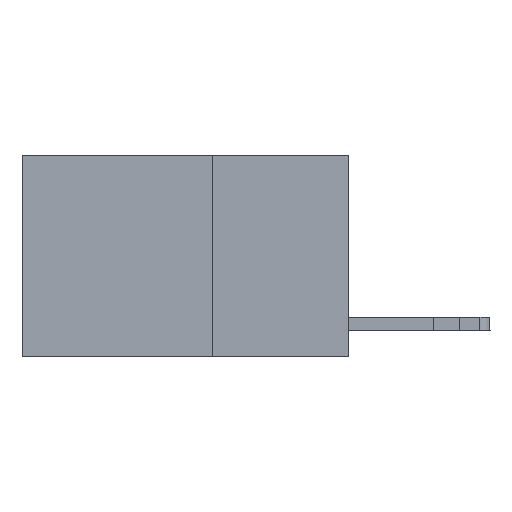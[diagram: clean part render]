
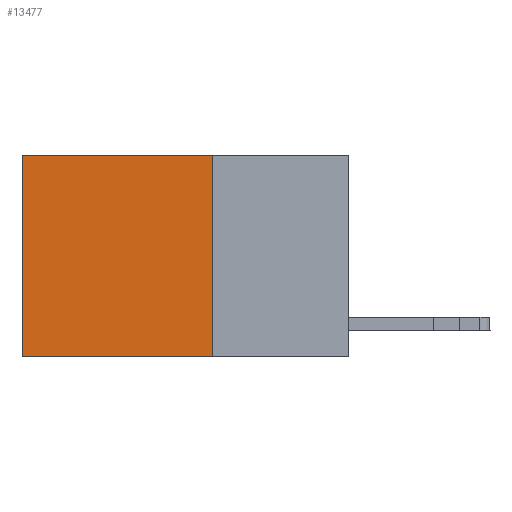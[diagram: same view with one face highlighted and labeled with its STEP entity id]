
A CAD part, left-side view. The second image highlights one B-rep face of the part: STEP entity #13477.
In plain terms, the highlighted planar face has unit normal (-1, 0, 0).
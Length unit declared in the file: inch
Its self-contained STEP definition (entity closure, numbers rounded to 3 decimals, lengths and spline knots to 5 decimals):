
#238 = CARTESIAN_POINT ( 'NONE',  ( 0.2625, 0.25, 0. ) ) ;
#240 = EDGE_CURVE ( 'NONE', #11728, #13563, #1599, .T. ) ;
#312 = DIRECTION ( 'NONE',  ( 0., 1., 0. ) ) ;
#482 = CARTESIAN_POINT ( 'NONE',  ( 0.2625, 0.6, 0. ) ) ;
#1485 = CARTESIAN_POINT ( 'NONE',  ( 0.2625, 0.25, -0.37 ) ) ;
#1599 = LINE ( 'NONE', #238, #4225 ) ;
#1971 = EDGE_LOOP ( 'NONE', ( #6994, #4688, #11610, #4409 ) ) ;
#4225 = VECTOR ( 'NONE', #13437, 39.37008 ) ;
#4297 = LINE ( 'NONE', #482, #6034 ) ;
#4409 = ORIENTED_EDGE ( 'NONE', *, *, #16206, .T. ) ;
#4688 = ORIENTED_EDGE ( 'NONE', *, *, #7152, .F. ) ;
#5557 = LINE ( 'NONE', #13019, #9569 ) ;
#5645 = DIRECTION ( 'NONE',  ( 0., 0., -1. ) ) ;
#6034 = VECTOR ( 'NONE', #5645, 39.37008 ) ;
#6400 = DIRECTION ( 'NONE',  ( 0., 0., -1. ) ) ;
#6994 = ORIENTED_EDGE ( 'NONE', *, *, #8410, .T. ) ;
#7145 = LINE ( 'NONE', #9414, #8613 ) ;
#7152 = EDGE_CURVE ( 'NONE', #13563, #13958, #5557, .T. ) ;
#7856 = CARTESIAN_POINT ( 'NONE',  ( 0.2625, 0.25, 0. ) ) ;
#8410 = EDGE_CURVE ( 'NONE', #10838, #13958, #4297, .T. ) ;
#8546 = CARTESIAN_POINT ( 'NONE',  ( 0.2625, 0.6, -0.37 ) ) ;
#8613 = VECTOR ( 'NONE', #14583, 39.37008 ) ;
#8931 = PLANE ( 'NONE',  #11508 ) ;
#9414 = CARTESIAN_POINT ( 'NONE',  ( 0.2625, 0.25, 0. ) ) ;
#9569 = VECTOR ( 'NONE', #312, 39.37008 ) ;
#10838 = VERTEX_POINT ( 'NONE', #16700 ) ;
#11467 = FACE_OUTER_BOUND ( 'NONE', #1971, .T. ) ;
#11508 = AXIS2_PLACEMENT_3D ( 'NONE', #14096, #16712, #6400 ) ;
#11610 = ORIENTED_EDGE ( 'NONE', *, *, #240, .F. ) ;
#11728 = VERTEX_POINT ( 'NONE', #7856 ) ;
#13019 = CARTESIAN_POINT ( 'NONE',  ( 0.2625, 0.25, -0.37 ) ) ;
#13437 = DIRECTION ( 'NONE',  ( 0., 0., -1. ) ) ;
#13477 = ADVANCED_FACE ( 'NONE', ( #11467 ), #8931, .F. ) ;
#13563 = VERTEX_POINT ( 'NONE', #1485 ) ;
#13958 = VERTEX_POINT ( 'NONE', #8546 ) ;
#14096 = CARTESIAN_POINT ( 'NONE',  ( 0.2625, 0.25, 0. ) ) ;
#14583 = DIRECTION ( 'NONE',  ( 0., 1., 0. ) ) ;
#16206 = EDGE_CURVE ( 'NONE', #11728, #10838, #7145, .T. ) ;
#16700 = CARTESIAN_POINT ( 'NONE',  ( 0.2625, 0.6, 0. ) ) ;
#16712 = DIRECTION ( 'NONE',  ( 1., 0., 0. ) ) ;
